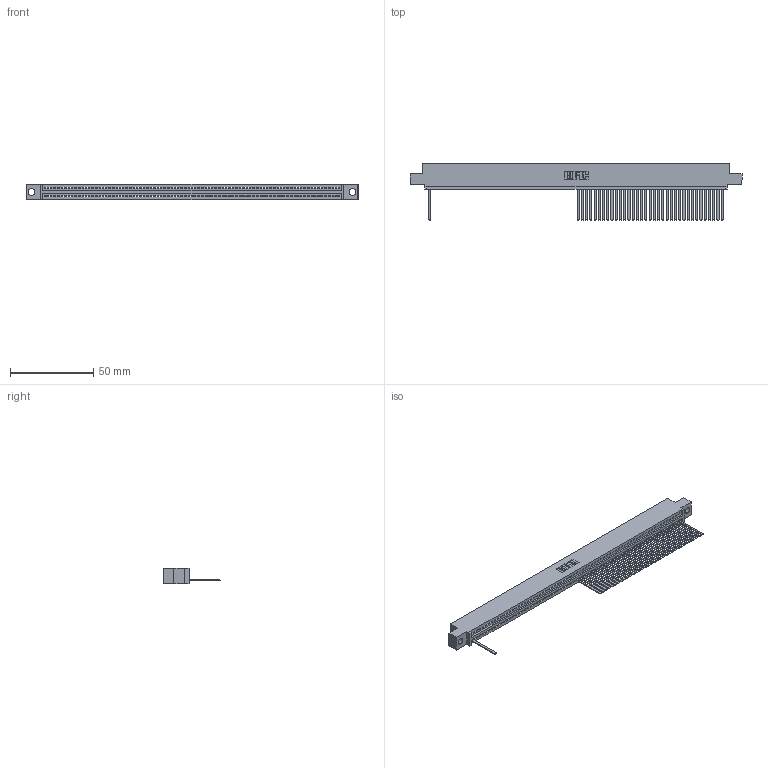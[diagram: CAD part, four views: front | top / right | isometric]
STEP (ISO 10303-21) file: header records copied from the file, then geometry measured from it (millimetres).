
FILE_DESCRIPTION (( 'STEP AP203' ), '1' );
FILE_NAME ('395-070-544-404.STEP', '2018-11-26T23:04:59', ( '' ), ( '' ), 'SwSTEP 2.0', 'SolidWorks 2016', '' );
FILE_SCHEMA (( 'CONFIG_CONTROL_DESIGN' ));
Length unit declared in the file: inch
Products named in the file (3): 345-292-001_345-293-144; 395-070-544-404; 345 Part_0.110 Offset - 0.156 Dia-TH
Assembly tree (37 placements, depth 2):
  395-070-544-404
    345 Part_0.110 Offset - 0.156 Dia-TH
    345-292-001_345-293-144  x36
Bounding box: 199.01 x 33.96 x 9.4 mm (x, y, z)
Volume: 18997.8 mm3; surface area: 24701.7 mm2
Topology: 37 solids, 37 shells, 2546 faces, 7877 edges, 5202 vertices
Faces by surface type: plane 1856, cylinder 690
Entity records: 47777 total; most frequent: ORIENTED_EDGE 8474, CARTESIAN_POINT 8436, DIRECTION 7285, EDGE_CURVE 4237, LINE 3829, VECTOR 3829, VERTEX_POINT 2822, AXIS2_PLACEMENT_3D 1728
